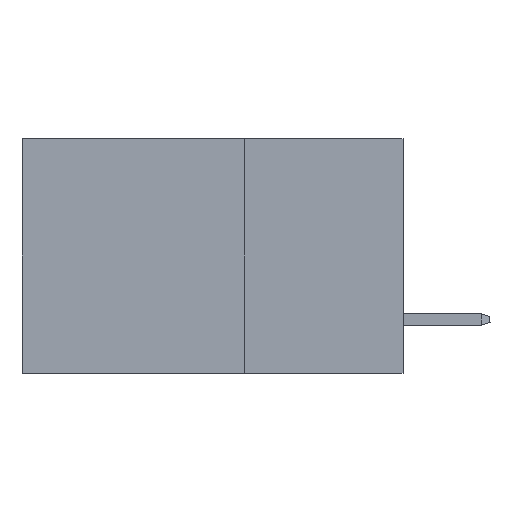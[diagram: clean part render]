
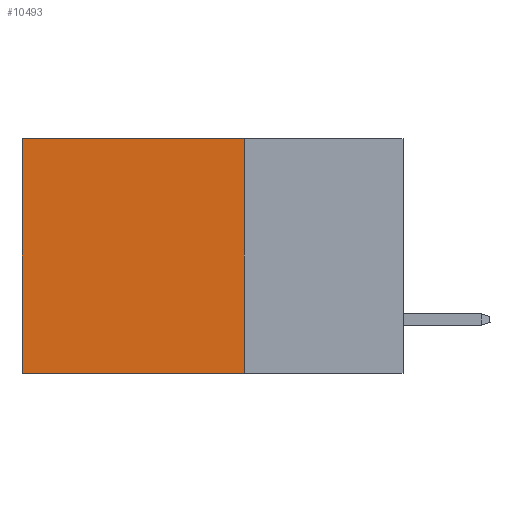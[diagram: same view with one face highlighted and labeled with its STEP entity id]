
A CAD part, left-side view. The second image highlights one B-rep face of the part: STEP entity #10493.
In plain terms, the highlighted planar face has unit normal (-1, 0, 0).
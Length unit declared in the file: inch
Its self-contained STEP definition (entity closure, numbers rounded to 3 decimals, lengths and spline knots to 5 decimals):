
#480 = EDGE_LOOP ( 'NONE', ( #11192, #17884, #14158, #2259 ) ) ;
#656 = VERTEX_POINT ( 'NONE', #5005 ) ;
#1194 = AXIS2_PLACEMENT_3D ( 'NONE', #5810, #2482, #13288 ) ;
#1367 = VECTOR ( 'NONE', #15190, 39.37008 ) ;
#1848 = DIRECTION ( 'NONE',  ( 0., 0., -1. ) ) ;
#2259 = ORIENTED_EDGE ( 'NONE', *, *, #8083, .T. ) ;
#2482 = DIRECTION ( 'NONE',  ( 1., 0., 0. ) ) ;
#3367 = VECTOR ( 'NONE', #9999, 39.37008 ) ;
#3674 = LINE ( 'NONE', #13230, #3367 ) ;
#4238 = PLANE ( 'NONE',  #1194 ) ;
#4969 = LINE ( 'NONE', #9631, #18918 ) ;
#5005 = CARTESIAN_POINT ( 'NONE',  ( 0.2875, 0.25, -0.37 ) ) ;
#5160 = CARTESIAN_POINT ( 'NONE',  ( 0.2875, 0.6, 0. ) ) ;
#5289 = DIRECTION ( 'NONE',  ( 0., 1., 0. ) ) ;
#5810 = CARTESIAN_POINT ( 'NONE',  ( 0.2875, 0.25, 0. ) ) ;
#6431 = VERTEX_POINT ( 'NONE', #18833 ) ;
#8083 = EDGE_CURVE ( 'NONE', #6431, #9632, #3674, .T. ) ;
#8367 = EDGE_CURVE ( 'NONE', #9632, #17191, #11870, .T. ) ;
#9153 = EDGE_CURVE ( 'NONE', #656, #17191, #14435, .T. ) ;
#9631 = CARTESIAN_POINT ( 'NONE',  ( 0.2875, 0.25, 0. ) ) ;
#9632 = VERTEX_POINT ( 'NONE', #19306 ) ;
#9855 = CARTESIAN_POINT ( 'NONE',  ( 0.2875, 0.25, -0.37 ) ) ;
#9999 = DIRECTION ( 'NONE',  ( 0., 1., 0. ) ) ;
#10493 = ADVANCED_FACE ( 'NONE', ( #13496 ), #4238, .F. ) ;
#11192 = ORIENTED_EDGE ( 'NONE', *, *, #8367, .T. ) ;
#11870 = LINE ( 'NONE', #5160, #1367 ) ;
#13230 = CARTESIAN_POINT ( 'NONE',  ( 0.2875, 0.25, 0. ) ) ;
#13288 = DIRECTION ( 'NONE',  ( 0., 0., -1. ) ) ;
#13496 = FACE_OUTER_BOUND ( 'NONE', #480, .T. ) ;
#14158 = ORIENTED_EDGE ( 'NONE', *, *, #15813, .F. ) ;
#14435 = LINE ( 'NONE', #9855, #19878 ) ;
#15190 = DIRECTION ( 'NONE',  ( 0., 0., -1. ) ) ;
#15813 = EDGE_CURVE ( 'NONE', #6431, #656, #4969, .T. ) ;
#16277 = CARTESIAN_POINT ( 'NONE',  ( 0.2875, 0.6, -0.37 ) ) ;
#17191 = VERTEX_POINT ( 'NONE', #16277 ) ;
#17884 = ORIENTED_EDGE ( 'NONE', *, *, #9153, .F. ) ;
#18833 = CARTESIAN_POINT ( 'NONE',  ( 0.2875, 0.25, 0. ) ) ;
#18918 = VECTOR ( 'NONE', #1848, 39.37008 ) ;
#19306 = CARTESIAN_POINT ( 'NONE',  ( 0.2875, 0.6, 0. ) ) ;
#19878 = VECTOR ( 'NONE', #5289, 39.37008 ) ;
